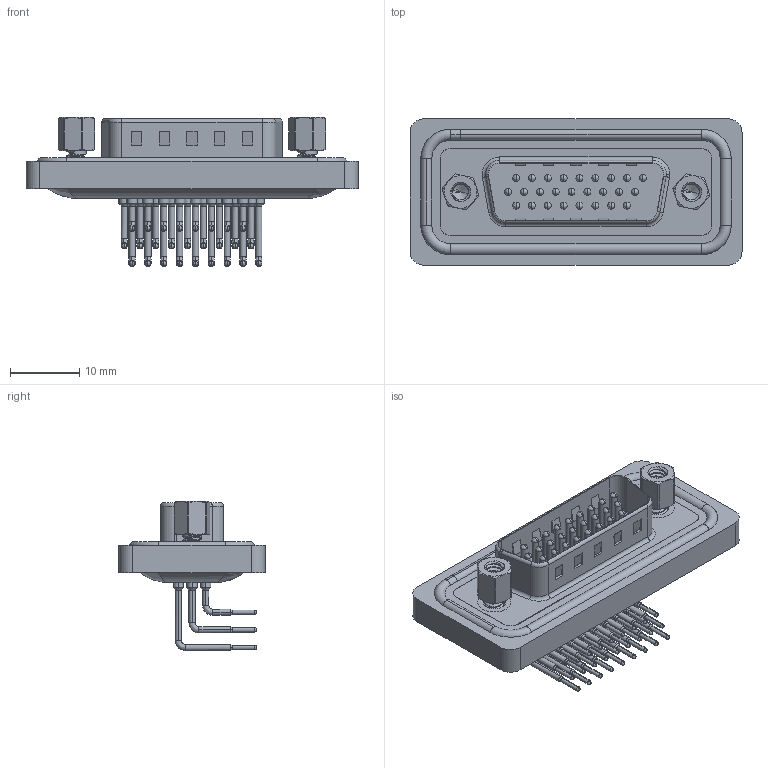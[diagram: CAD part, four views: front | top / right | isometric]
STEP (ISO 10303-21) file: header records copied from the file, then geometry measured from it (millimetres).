
FILE_DESCRIPTION (( 'STEP AP203' ), '1' );
FILE_NAME ('633-W26-662-012.STEP', '2024-04-12T18:34:43', ( '' ), ( '' ), 'SwSTEP 2.0', 'SolidWorks 2023', '' );
FILE_SCHEMA (( 'CONFIG_CONTROL_DESIGN' ));
Length unit declared in the file: millimetre
Products named in the file (9): 633W 4-40 Hex Standoff; 633W Housing_26 Contacts; 633W 4-40 Threaded Rivet_Stabilizer; 633W Waterproof Housing_26 Contacts; 633W Contact Row 2; 633-W26-662-012; 633W Contact Row 3; 633W Contact Row 1; 633W Shell_26 Contacts
Assembly tree (33 placements, depth 2):
  633-W26-662-012
    633W Housing_26 Contacts
    633W Shell_26 Contacts
    633W Waterproof Housing_26 Contacts
    633W Contact Row 1  x9
    633W Contact Row 2  x9
    633W Contact Row 3  x8
    633W 4-40 Threaded Rivet_Stabilizer  x2
    633W 4-40 Hex Standoff  x2
Bounding box: 47.89 x 21.1 x 21.52 mm (x, y, z)
Volume: 5051.7 mm3; surface area: 9687.1 mm2
Topology: 34 solids, 34 shells, 3388 faces, 9464 edges, 6155 vertices
Faces by surface type: plane 1837, cylinder 1198, bspline 178, cone 132, torus 43
Entity records: 35329 total; most frequent: CARTESIAN_POINT 9609, DIRECTION 5193, ORIENTED_EDGE 4938, EDGE_CURVE 2469, AXIS2_PLACEMENT_3D 1908, VERTEX_POINT 1611, LINE 1377, VECTOR 1377
